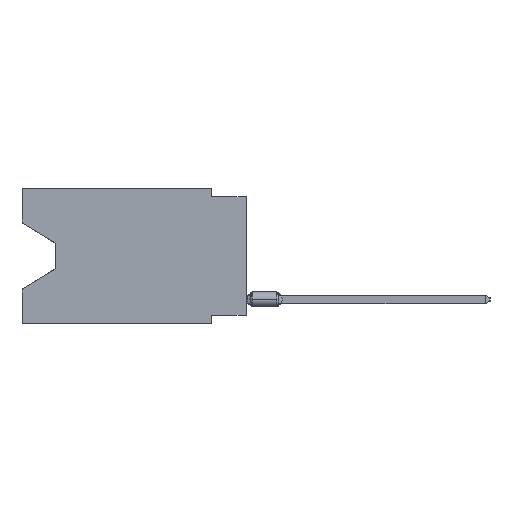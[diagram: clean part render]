
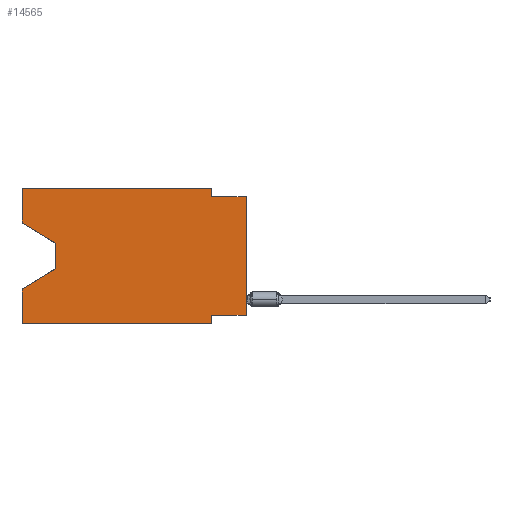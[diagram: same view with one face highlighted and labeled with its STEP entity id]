
A CAD part, left-side view. The second image highlights one B-rep face of the part: STEP entity #14565.
In plain terms, the highlighted planar face has unit normal (-1, 0, 0).
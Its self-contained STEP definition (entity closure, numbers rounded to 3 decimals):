
#589 = EDGE_CURVE ( 'NONE', #18700, #5609, #28266, .T. ) ;
#745 = LINE ( 'NONE', #9662, #7207 ) ;
#916 = VECTOR ( 'NONE', #30141, 1000. ) ;
#955 = CARTESIAN_POINT ( 'NONE',  ( 0., 0., -9.271 ) ) ;
#1661 = CARTESIAN_POINT ( 'NONE',  ( 0., 16.383, -2.546 ) ) ;
#2141 = CARTESIAN_POINT ( 'NONE',  ( 0., 2.54, -9.906 ) ) ;
#2270 = LINE ( 'NONE', #10429, #22849 ) ;
#3818 = PLANE ( 'NONE',  #35719 ) ;
#3877 = EDGE_CURVE ( 'NONE', #22890, #23984, #5048, .T. ) ;
#4858 = ORIENTED_EDGE ( 'NONE', *, *, #34354, .F. ) ;
#5048 = LINE ( 'NONE', #28151, #18668 ) ;
#5099 = DIRECTION ( 'NONE',  ( 0., 0., 1. ) ) ;
#5262 = CARTESIAN_POINT ( 'NONE',  ( 0., 16.383, 0. ) ) ;
#5576 = ORIENTED_EDGE ( 'NONE', *, *, #24184, .F. ) ;
#5609 = VERTEX_POINT ( 'NONE', #24189 ) ;
#6297 = CARTESIAN_POINT ( 'NONE',  ( 0., 13.97, -4.013 ) ) ;
#6833 = CARTESIAN_POINT ( 'NONE',  ( 0., 13.97, -5.893 ) ) ;
#7201 = CARTESIAN_POINT ( 'NONE',  ( 0., 2.54, -9.906 ) ) ;
#7207 = VECTOR ( 'NONE', #18567, 1000. ) ;
#7554 = CARTESIAN_POINT ( 'NONE',  ( 0., 16.383, -7.36 ) ) ;
#7864 = CARTESIAN_POINT ( 'NONE',  ( 0., 16.383, 0. ) ) ;
#7888 = VECTOR ( 'NONE', #21323, 1000. ) ;
#7937 = CARTESIAN_POINT ( 'NONE',  ( 0., 16.383, 0. ) ) ;
#8762 = CARTESIAN_POINT ( 'NONE',  ( 0., 16.383, 0. ) ) ;
#9038 = CARTESIAN_POINT ( 'NONE',  ( 0., 16.383, -9.906 ) ) ;
#9321 = CARTESIAN_POINT ( 'NONE',  ( 0., 2.54, -9.271 ) ) ;
#9662 = CARTESIAN_POINT ( 'NONE',  ( 0., 0., 0. ) ) ;
#10429 = CARTESIAN_POINT ( 'NONE',  ( 0., 0., -0.635 ) ) ;
#10546 = VECTOR ( 'NONE', #19981, 1000. ) ;
#10730 = ORIENTED_EDGE ( 'NONE', *, *, #589, .F. ) ;
#11249 = VERTEX_POINT ( 'NONE', #20071 ) ;
#11322 = DIRECTION ( 'NONE',  ( 0., 0., 1. ) ) ;
#12537 = CARTESIAN_POINT ( 'NONE',  ( 0., 16.383, 0. ) ) ;
#13173 = ORIENTED_EDGE ( 'NONE', *, *, #19420, .F. ) ;
#13436 = LINE ( 'NONE', #16100, #28284 ) ;
#14565 = ADVANCED_FACE ( 'NONE', ( #35643 ), #3818, .F. ) ;
#14607 = EDGE_CURVE ( 'NONE', #31310, #37027, #27110, .T. ) ;
#14890 = VERTEX_POINT ( 'NONE', #31879 ) ;
#15000 = LINE ( 'NONE', #28821, #17255 ) ;
#15198 = CARTESIAN_POINT ( 'NONE',  ( 0., 13.97, -5.893 ) ) ;
#16100 = CARTESIAN_POINT ( 'NONE',  ( 0., 13.97, -4.013 ) ) ;
#16619 = ORIENTED_EDGE ( 'NONE', *, *, #36883, .T. ) ;
#17255 = VECTOR ( 'NONE', #20864, 1000. ) ;
#17791 = ORIENTED_EDGE ( 'NONE', *, *, #18278, .F. ) ;
#18278 = EDGE_CURVE ( 'NONE', #14890, #11249, #2270, .T. ) ;
#18567 = DIRECTION ( 'NONE',  ( 0., 0., 1. ) ) ;
#18668 = VECTOR ( 'NONE', #31381, 1000. ) ;
#18700 = VERTEX_POINT ( 'NONE', #7864 ) ;
#18946 = DIRECTION ( 'NONE',  ( 0., 0., -1. ) ) ;
#19157 = DIRECTION ( 'NONE',  ( 0., -1., 0. ) ) ;
#19420 = EDGE_CURVE ( 'NONE', #22890, #18700, #19478, .T. ) ;
#19478 = LINE ( 'NONE', #5262, #35178 ) ;
#19981 = DIRECTION ( 'NONE',  ( 0., 0., -1. ) ) ;
#20071 = CARTESIAN_POINT ( 'NONE',  ( 0., 0., -0.635 ) ) ;
#20864 = DIRECTION ( 'NONE',  ( 0., -1., 0. ) ) ;
#20879 = LINE ( 'NONE', #15198, #916 ) ;
#21073 = DIRECTION ( 'NONE',  ( 0., 1., 0. ) ) ;
#21323 = DIRECTION ( 'NONE',  ( 0., 0., -1. ) ) ;
#21685 = EDGE_CURVE ( 'NONE', #31310, #11249, #745, .T. ) ;
#22464 = EDGE_LOOP ( 'NONE', ( #32161, #27849, #16619, #5576, #25386, #30117, #29049, #28918, #17791, #4858, #10730, #13173 ) ) ;
#22585 = DIRECTION ( 'NONE',  ( 0., -1., 0. ) ) ;
#22849 = VECTOR ( 'NONE', #19157, 1000. ) ;
#22890 = VERTEX_POINT ( 'NONE', #1661 ) ;
#23897 = CARTESIAN_POINT ( 'NONE',  ( 0., 0., -9.271 ) ) ;
#23984 = VERTEX_POINT ( 'NONE', #6297 ) ;
#24096 = DIRECTION ( 'NONE',  ( 0., 0., -1. ) ) ;
#24184 = EDGE_CURVE ( 'NONE', #28232, #30256, #28010, .T. ) ;
#24189 = CARTESIAN_POINT ( 'NONE',  ( 0., 2.54, 0. ) ) ;
#24708 = LINE ( 'NONE', #36256, #7888 ) ;
#25386 = ORIENTED_EDGE ( 'NONE', *, *, #29010, .T. ) ;
#25803 = VECTOR ( 'NONE', #22585, 1000. ) ;
#26345 = DIRECTION ( 'NONE',  ( 1., 0., 0. ) ) ;
#27110 = LINE ( 'NONE', #23897, #32084 ) ;
#27849 = ORIENTED_EDGE ( 'NONE', *, *, #35819, .T. ) ;
#28010 = LINE ( 'NONE', #7937, #32366 ) ;
#28151 = CARTESIAN_POINT ( 'NONE',  ( 0., 16.383, -2.546 ) ) ;
#28232 = VERTEX_POINT ( 'NONE', #9038 ) ;
#28266 = LINE ( 'NONE', #8762, #25803 ) ;
#28284 = VECTOR ( 'NONE', #18946, 1000. ) ;
#28509 = EDGE_CURVE ( 'NONE', #37027, #29147, #36990, .T. ) ;
#28821 = CARTESIAN_POINT ( 'NONE',  ( 0., 16.383, -9.906 ) ) ;
#28918 = ORIENTED_EDGE ( 'NONE', *, *, #21685, .T. ) ;
#29010 = EDGE_CURVE ( 'NONE', #28232, #29147, #15000, .T. ) ;
#29049 = ORIENTED_EDGE ( 'NONE', *, *, #14607, .F. ) ;
#29147 = VERTEX_POINT ( 'NONE', #7201 ) ;
#30117 = ORIENTED_EDGE ( 'NONE', *, *, #28509, .F. ) ;
#30141 = DIRECTION ( 'NONE',  ( 0., 0.855, -0.519 ) ) ;
#30256 = VERTEX_POINT ( 'NONE', #7554 ) ;
#31310 = VERTEX_POINT ( 'NONE', #955 ) ;
#31381 = DIRECTION ( 'NONE',  ( 0., -0.855, -0.519 ) ) ;
#31879 = CARTESIAN_POINT ( 'NONE',  ( 0., 2.54, -0.635 ) ) ;
#32084 = VECTOR ( 'NONE', #21073, 1000. ) ;
#32161 = ORIENTED_EDGE ( 'NONE', *, *, #3877, .T. ) ;
#32366 = VECTOR ( 'NONE', #5099, 1000. ) ;
#34354 = EDGE_CURVE ( 'NONE', #5609, #14890, #24708, .T. ) ;
#35100 = VERTEX_POINT ( 'NONE', #6833 ) ;
#35178 = VECTOR ( 'NONE', #11322, 1000. ) ;
#35643 = FACE_OUTER_BOUND ( 'NONE', #22464, .T. ) ;
#35719 = AXIS2_PLACEMENT_3D ( 'NONE', #12537, #26345, #24096 ) ;
#35819 = EDGE_CURVE ( 'NONE', #23984, #35100, #13436, .T. ) ;
#36256 = CARTESIAN_POINT ( 'NONE',  ( 0., 2.54, 0. ) ) ;
#36883 = EDGE_CURVE ( 'NONE', #35100, #30256, #20879, .T. ) ;
#36990 = LINE ( 'NONE', #2141, #10546 ) ;
#37027 = VERTEX_POINT ( 'NONE', #9321 ) ;
